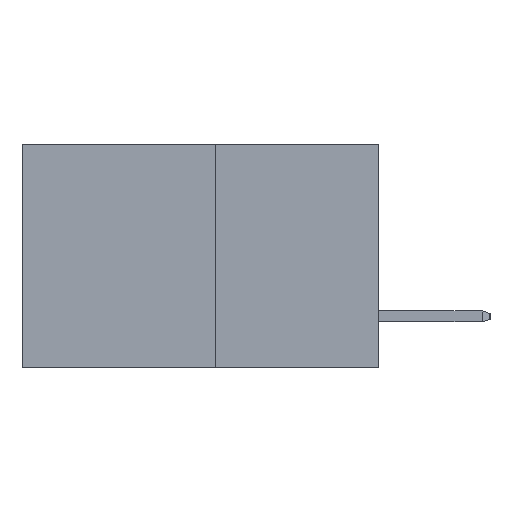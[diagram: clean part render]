
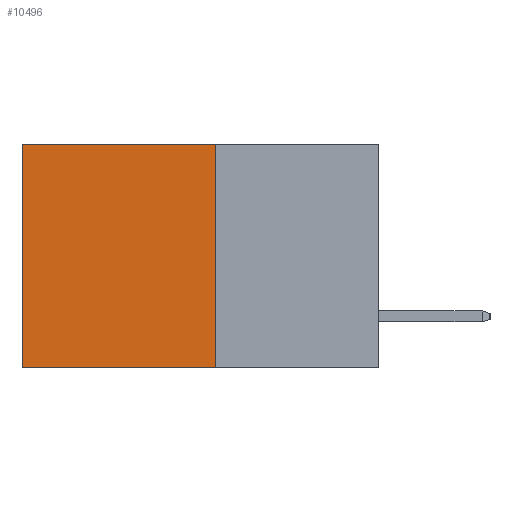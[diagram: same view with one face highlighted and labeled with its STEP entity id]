
A CAD part, left-side view. The second image highlights one B-rep face of the part: STEP entity #10496.
In plain terms, the highlighted planar face has unit normal (-1, 0, 0).
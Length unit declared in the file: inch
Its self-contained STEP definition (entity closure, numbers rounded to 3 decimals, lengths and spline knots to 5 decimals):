
#1089 = VERTEX_POINT ( 'NONE', #2195 ) ;
#1309 = AXIS2_PLACEMENT_3D ( 'NONE', #7393, #9782, #4866 ) ;
#2194 = VERTEX_POINT ( 'NONE', #9545 ) ;
#2195 = CARTESIAN_POINT ( 'NONE',  ( 0.277, 0.59, -0.37 ) ) ;
#2428 = VECTOR ( 'NONE', #5450, 39.37008 ) ;
#2609 = CARTESIAN_POINT ( 'NONE',  ( 0.277, 0.27, -0.37 ) ) ;
#2758 = VERTEX_POINT ( 'NONE', #10046 ) ;
#2896 = EDGE_CURVE ( 'NONE', #2194, #1089, #9340, .T. ) ;
#3269 = ORIENTED_EDGE ( 'NONE', *, *, #6667, .F. ) ;
#4191 = LINE ( 'NONE', #4552, #2428 ) ;
#4471 = ORIENTED_EDGE ( 'NONE', *, *, #7955, .F. ) ;
#4552 = CARTESIAN_POINT ( 'NONE',  ( 0.277, 0.27, -0.37 ) ) ;
#4687 = LINE ( 'NONE', #9496, #6710 ) ;
#4720 = EDGE_LOOP ( 'NONE', ( #6239, #3269, #4471, #6438 ) ) ;
#4852 = VERTEX_POINT ( 'NONE', #2609 ) ;
#4866 = DIRECTION ( 'NONE',  ( 0., 0., -1. ) ) ;
#5450 = DIRECTION ( 'NONE',  ( 0., 1., 0. ) ) ;
#5550 = FACE_OUTER_BOUND ( 'NONE', #4720, .T. ) ;
#5922 = DIRECTION ( 'NONE',  ( 0., 1., 0. ) ) ;
#6239 = ORIENTED_EDGE ( 'NONE', *, *, #2896, .T. ) ;
#6438 = ORIENTED_EDGE ( 'NONE', *, *, #10057, .T. ) ;
#6531 = LINE ( 'NONE', #9213, #8712 ) ;
#6667 = EDGE_CURVE ( 'NONE', #4852, #1089, #4191, .T. ) ;
#6710 = VECTOR ( 'NONE', #7096, 39.37008 ) ;
#7096 = DIRECTION ( 'NONE',  ( 0., 0., -1. ) ) ;
#7387 = DIRECTION ( 'NONE',  ( 0., 0., -1. ) ) ;
#7393 = CARTESIAN_POINT ( 'NONE',  ( 0.277, 0.27, -0.37 ) ) ;
#7955 = EDGE_CURVE ( 'NONE', #2758, #4852, #4687, .T. ) ;
#8189 = PLANE ( 'NONE',  #1309 ) ;
#8534 = CARTESIAN_POINT ( 'NONE',  ( 0.277, 0.59, -0.37 ) ) ;
#8562 = VECTOR ( 'NONE', #7387, 39.37008 ) ;
#8712 = VECTOR ( 'NONE', #5922, 39.37008 ) ;
#9213 = CARTESIAN_POINT ( 'NONE',  ( 0.277, 0.27, 0. ) ) ;
#9340 = LINE ( 'NONE', #8534, #8562 ) ;
#9496 = CARTESIAN_POINT ( 'NONE',  ( 0.277, 0.27, -0.37 ) ) ;
#9545 = CARTESIAN_POINT ( 'NONE',  ( 0.277, 0.59, 0. ) ) ;
#9782 = DIRECTION ( 'NONE',  ( 1., 0., 0. ) ) ;
#10046 = CARTESIAN_POINT ( 'NONE',  ( 0.277, 0.27, 0. ) ) ;
#10057 = EDGE_CURVE ( 'NONE', #2758, #2194, #6531, .T. ) ;
#10496 = ADVANCED_FACE ( 'NONE', ( #5550 ), #8189, .F. ) ;
